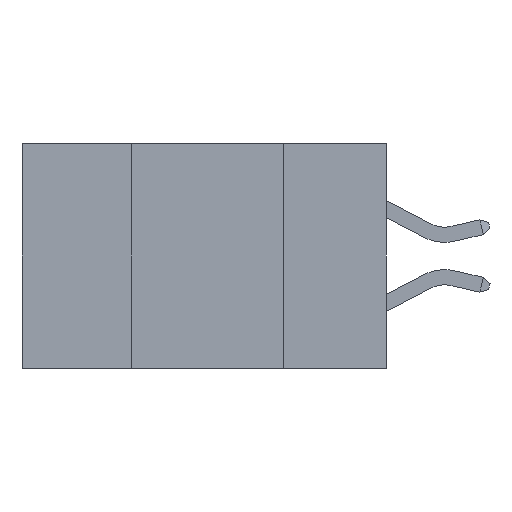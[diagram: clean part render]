
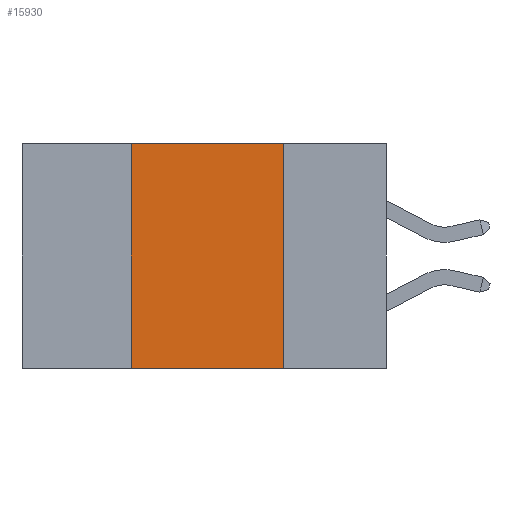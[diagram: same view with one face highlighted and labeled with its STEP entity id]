
A CAD part, left-side view. The second image highlights one B-rep face of the part: STEP entity #15930.
In plain terms, the highlighted planar face has unit normal (-1, 0, 0).
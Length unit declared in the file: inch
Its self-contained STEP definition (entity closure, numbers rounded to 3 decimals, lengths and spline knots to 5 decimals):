
#3 = EDGE_CURVE ( 'NONE', #14099, #6043, #1434, .T. ) ;
#171 = EDGE_LOOP ( 'NONE', ( #8423, #6182, #6603, #13718 ) ) ;
#429 = DIRECTION ( 'NONE',  ( 0., 0., 1. ) ) ;
#778 = CARTESIAN_POINT ( 'NONE',  ( 0., 0.17, -0.37 ) ) ;
#955 = EDGE_CURVE ( 'NONE', #6043, #5982, #17521, .T. ) ;
#1329 = CARTESIAN_POINT ( 'NONE',  ( 0., 0.42, -0.37 ) ) ;
#1434 = LINE ( 'NONE', #9277, #15472 ) ;
#1661 = LINE ( 'NONE', #12741, #4519 ) ;
#2879 = CARTESIAN_POINT ( 'NONE',  ( 0., 0.6, 0. ) ) ;
#4144 = CARTESIAN_POINT ( 'NONE',  ( 0., 0.6, -0.37 ) ) ;
#4519 = VECTOR ( 'NONE', #429, 39.37008 ) ;
#4553 = VECTOR ( 'NONE', #6957, 39.37008 ) ;
#4712 = VERTEX_POINT ( 'NONE', #1329 ) ;
#5982 = VERTEX_POINT ( 'NONE', #778 ) ;
#6043 = VERTEX_POINT ( 'NONE', #15824 ) ;
#6182 = ORIENTED_EDGE ( 'NONE', *, *, #3, .F. ) ;
#6603 = ORIENTED_EDGE ( 'NONE', *, *, #16783, .F. ) ;
#6957 = DIRECTION ( 'NONE',  ( 0., -1., 0. ) ) ;
#7080 = DIRECTION ( 'NONE',  ( 0., 0., -1. ) ) ;
#8423 = ORIENTED_EDGE ( 'NONE', *, *, #955, .F. ) ;
#8643 = LINE ( 'NONE', #4144, #4553 ) ;
#9277 = CARTESIAN_POINT ( 'NONE',  ( 0., 0.6, 0. ) ) ;
#9620 = VECTOR ( 'NONE', #9978, 39.37008 ) ;
#9978 = DIRECTION ( 'NONE',  ( 0., 0., -1. ) ) ;
#10730 = AXIS2_PLACEMENT_3D ( 'NONE', #2879, #15059, #7080 ) ;
#12741 = CARTESIAN_POINT ( 'NONE',  ( 0., 0.42, -0.37 ) ) ;
#13682 = PLANE ( 'NONE',  #10730 ) ;
#13718 = ORIENTED_EDGE ( 'NONE', *, *, #15887, .T. ) ;
#14099 = VERTEX_POINT ( 'NONE', #16516 ) ;
#14472 = FACE_OUTER_BOUND ( 'NONE', #171, .T. ) ;
#15059 = DIRECTION ( 'NONE',  ( 1., 0., 0. ) ) ;
#15472 = VECTOR ( 'NONE', #17494, 39.37008 ) ;
#15824 = CARTESIAN_POINT ( 'NONE',  ( 0., 0.17, 0. ) ) ;
#15887 = EDGE_CURVE ( 'NONE', #4712, #5982, #8643, .T. ) ;
#15930 = ADVANCED_FACE ( 'NONE', ( #14472 ), #13682, .F. ) ;
#16048 = CARTESIAN_POINT ( 'NONE',  ( 0., 0.17, -0.37 ) ) ;
#16516 = CARTESIAN_POINT ( 'NONE',  ( 0., 0.42, 0. ) ) ;
#16783 = EDGE_CURVE ( 'NONE', #4712, #14099, #1661, .T. ) ;
#17494 = DIRECTION ( 'NONE',  ( 0., -1., 0. ) ) ;
#17521 = LINE ( 'NONE', #16048, #9620 ) ;
